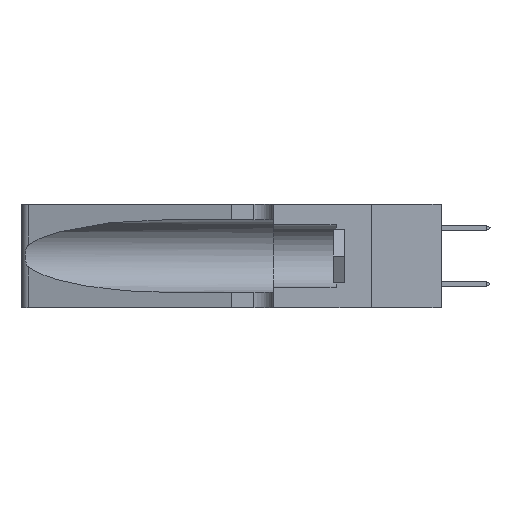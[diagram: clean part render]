
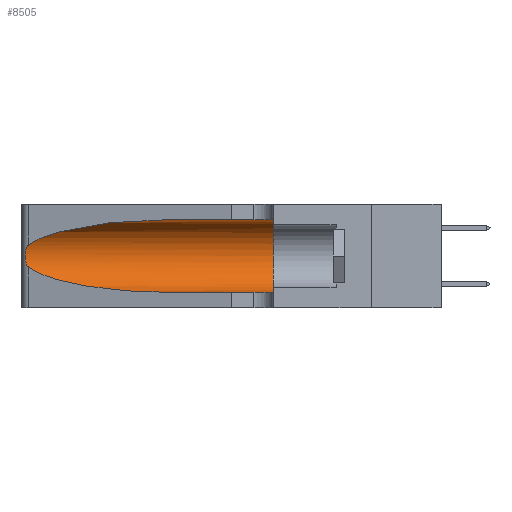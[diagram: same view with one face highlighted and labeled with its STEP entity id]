
A CAD part, left-side view. The second image highlights one B-rep face of the part: STEP entity #8505.
In plain terms, the highlighted cylindrical face has radius 3.308 mm (diameter 6.617 mm), a partial arc.
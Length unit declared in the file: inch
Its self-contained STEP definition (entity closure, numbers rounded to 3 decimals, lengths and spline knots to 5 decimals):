
#109 = DIRECTION ( 'NONE',  ( 0., 1., 0. ) ) ;
#704 = LINE ( 'NONE', #2474, #22109 ) ;
#752 = AXIS2_PLACEMENT_3D ( 'NONE', #15760, #17824, #25936 ) ;
#983 = VERTEX_POINT ( 'NONE', #8252 ) ;
#1059 = B_SPLINE_CURVE_WITH_KNOTS ( 'NONE', 3,
 ( #11884, #7702, #24182, #13987, #1482, #16075, #3581, #18135, #5696, #20170, #7795, #22230, #9864, #24276 ),
 .UNSPECIFIED., .F., .F.,
 ( 4, 2, 2, 2, 2, 2, 4 ),
 ( 0., 0.00027, 0.00053, 0.00107, 0.0016, 0.00187, 0.00214 ),
 .UNSPECIFIED. ) ;
#1482 = CARTESIAN_POINT ( 'NONE',  ( 0.25854, 1.2359, 0.20912 ) ) ;
#1843 = AXIS2_PLACEMENT_3D ( 'NONE', #12598, #109, #14698 ) ;
#2376 = CARTESIAN_POINT ( 'NONE',  ( 0.1305, 0.72297, 0.31525 ) ) ;
#2474 = CARTESIAN_POINT ( 'NONE',  ( 0.1305, 1.61858, 0.05475 ) ) ;
#3581 = CARTESIAN_POINT ( 'NONE',  ( 0.26075, 1.23896, 0.19203 ) ) ;
#3908 =( BOUNDED_CURVE ( )  B_SPLINE_CURVE ( 3, ( #19160, #6661, #21192, #8821 ),
 .UNSPECIFIED., .F., .T. ) 
 B_SPLINE_CURVE_WITH_KNOTS ( ( 4, 4 ),
 ( 3.44316, 4.71239 ),
 .UNSPECIFIED. ) 
 CURVE ( )  GEOMETRIC_REPRESENTATION_ITEM ( )  RATIONAL_B_SPLINE_CURVE ( ( 1., 0.87, 0.87, 1. ) ) 
 REPRESENTATION_ITEM ( '' )  );
#4470 = CARTESIAN_POINT ( 'NONE',  ( 0.2373, 1.15595, 0.28018 ) ) ;
#5696 = CARTESIAN_POINT ( 'NONE',  ( 0.26017, 1.23833, 0.17102 ) ) ;
#5847 = VERTEX_POINT ( 'NONE', #11163 ) ;
#6070 = EDGE_CURVE ( 'NONE', #23012, #17905, #1059, .T. ) ;
#6661 = CARTESIAN_POINT ( 'NONE',  ( 0.2373, 1.15595, 0.08982 ) ) ;
#6668 = EDGE_LOOP ( 'NONE', ( #10275, #7941, #16881, #20737, #11361, #8918 ) ) ;
#7315 = CARTESIAN_POINT ( 'NONE',  ( 0.1305, 0.72297, 0.31525 ) ) ;
#7702 = CARTESIAN_POINT ( 'NONE',  ( 0.25555, 1.22994, 0.2215 ) ) ;
#7795 = CARTESIAN_POINT ( 'NONE',  ( 0.25789, 1.23486, 0.15765 ) ) ;
#7941 = ORIENTED_EDGE ( 'NONE', *, *, #6070, .T. ) ;
#7994 = CARTESIAN_POINT ( 'NONE',  ( 0.25487, 1.22718, 0.22369 ) ) ;
#8252 = CARTESIAN_POINT ( 'NONE',  ( 0.1305, 0.35, 0.05475 ) ) ;
#8505 = ADVANCED_FACE ( 'NONE', ( #22934 ), #11359, .F. ) ;
#8508 = CARTESIAN_POINT ( 'NONE',  ( 0.1305, 1.61858, 0.31525 ) ) ;
#8691 = VERTEX_POINT ( 'NONE', #10106 ) ;
#8821 = CARTESIAN_POINT ( 'NONE',  ( 0.1305, 0.72297, 0.05475 ) ) ;
#8918 = ORIENTED_EDGE ( 'NONE', *, *, #23159, .F. ) ;
#9864 = CARTESIAN_POINT ( 'NONE',  ( 0.25555, 1.22993, 0.14849 ) ) ;
#10106 = CARTESIAN_POINT ( 'NONE',  ( 0.1305, 0.72297, 0.05475 ) ) ;
#10275 = ORIENTED_EDGE ( 'NONE', *, *, #17228, .T. ) ;
#10539 = EDGE_CURVE ( 'NONE', #5847, #983, #17742, .T. ) ;
#10778 = DIRECTION ( 'NONE',  ( 0., -1., 0. ) ) ;
#10884 = VERTEX_POINT ( 'NONE', #7315 ) ;
#11163 = CARTESIAN_POINT ( 'NONE',  ( 0.1305, 0.35, 0.31525 ) ) ;
#11359 = CYLINDRICAL_SURFACE ( 'NONE', #752, 0.13025 ) ;
#11361 = ORIENTED_EDGE ( 'NONE', *, *, #10539, .F. ) ;
#11601 =( BOUNDED_CURVE ( )  B_SPLINE_CURVE ( 3, ( #2376, #14856, #4470, #18994 ),
 .UNSPECIFIED., .F., .T. ) 
 B_SPLINE_CURVE_WITH_KNOTS ( ( 4, 4 ),
 ( 1.5708, 2.84003 ),
 .UNSPECIFIED. ) 
 CURVE ( )  GEOMETRIC_REPRESENTATION_ITEM ( )  RATIONAL_B_SPLINE_CURVE ( ( 1., 0.87, 0.87, 1. ) ) 
 REPRESENTATION_ITEM ( '' )  );
#11884 = CARTESIAN_POINT ( 'NONE',  ( 0.25487, 1.22718, 0.22369 ) ) ;
#12598 = CARTESIAN_POINT ( 'NONE',  ( 0.1305, 0.35, 0.185 ) ) ;
#12706 = EDGE_CURVE ( 'NONE', #8691, #983, #704, .T. ) ;
#13987 = CARTESIAN_POINT ( 'NONE',  ( 0.25787, 1.23484, 0.2124 ) ) ;
#14241 = VECTOR ( 'NONE', #22944, 39.37008 ) ;
#14520 = EDGE_CURVE ( 'NONE', #17905, #8691, #3908, .T. ) ;
#14698 = DIRECTION ( 'NONE',  ( 0., 0., 1. ) ) ;
#14856 = CARTESIAN_POINT ( 'NONE',  ( 0.18966, 0.96281, 0.31525 ) ) ;
#15760 = CARTESIAN_POINT ( 'NONE',  ( 0.1305, 1.61858, 0.185 ) ) ;
#16075 = CARTESIAN_POINT ( 'NONE',  ( 0.26018, 1.23835, 0.19895 ) ) ;
#16881 = ORIENTED_EDGE ( 'NONE', *, *, #14520, .T. ) ;
#17084 = CARTESIAN_POINT ( 'NONE',  ( 0.25487, 1.22718, 0.14631 ) ) ;
#17228 = EDGE_CURVE ( 'NONE', #10884, #23012, #11601, .T. ) ;
#17742 = CIRCLE ( 'NONE', #1843, 0.13025 ) ;
#17824 = DIRECTION ( 'NONE',  ( 0., -1., 0. ) ) ;
#17905 = VERTEX_POINT ( 'NONE', #17084 ) ;
#18135 = CARTESIAN_POINT ( 'NONE',  ( 0.26075, 1.23896, 0.178 ) ) ;
#18994 = CARTESIAN_POINT ( 'NONE',  ( 0.25487, 1.22718, 0.22369 ) ) ;
#19058 = LINE ( 'NONE', #8508, #14241 ) ;
#19160 = CARTESIAN_POINT ( 'NONE',  ( 0.25487, 1.22718, 0.14631 ) ) ;
#20170 = CARTESIAN_POINT ( 'NONE',  ( 0.25856, 1.23593, 0.16098 ) ) ;
#20737 = ORIENTED_EDGE ( 'NONE', *, *, #12706, .T. ) ;
#21192 = CARTESIAN_POINT ( 'NONE',  ( 0.18966, 0.96281, 0.05475 ) ) ;
#22109 = VECTOR ( 'NONE', #10778, 39.37008 ) ;
#22230 = CARTESIAN_POINT ( 'NONE',  ( 0.25639, 1.23186, 0.15144 ) ) ;
#22934 = FACE_OUTER_BOUND ( 'NONE', #6668, .T. ) ;
#22944 = DIRECTION ( 'NONE',  ( 0., -1., 0. ) ) ;
#23012 = VERTEX_POINT ( 'NONE', #7994 ) ;
#23159 = EDGE_CURVE ( 'NONE', #10884, #5847, #19058, .T. ) ;
#24182 = CARTESIAN_POINT ( 'NONE',  ( 0.25639, 1.23184, 0.21858 ) ) ;
#24276 = CARTESIAN_POINT ( 'NONE',  ( 0.25487, 1.22718, 0.14631 ) ) ;
#25936 = DIRECTION ( 'NONE',  ( 0., 0., -1. ) ) ;
